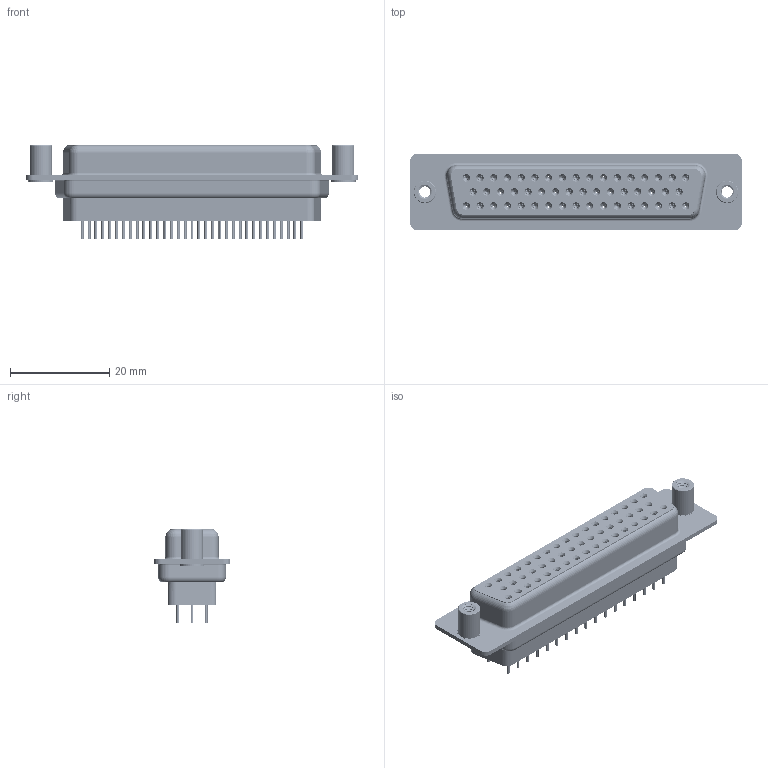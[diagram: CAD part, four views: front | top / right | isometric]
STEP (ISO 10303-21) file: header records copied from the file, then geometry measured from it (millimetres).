
FILE_DESCRIPTION (( 'STEP AP203' ), '1' );
FILE_NAME ('628-050-228-268.STEP', '2020-07-21T01:35:46', ( '' ), ( '' ), 'SwSTEP 2.0', 'SolidWorks 2020', '' );
FILE_SCHEMA (( 'CONFIG_CONTROL_DESIGN' ));
Length unit declared in the file: millimetre
Products named in the file (8): 628 4-40 Threaded Standoff; 628 Contact Row 1_28L; 628 Housing_50 FF; 628 Contact Row 2_28L; 628 Shell Front_50 Contacts; 628 Shell Rear_50 Contacts; 628-050-228-268; 628 Contact Row 3_28L
Assembly tree (55 placements, depth 2):
  628-050-228-268
    628 Housing_50 FF
    628 Shell Front_50 Contacts
    628 Shell Rear_50 Contacts
    628 Contact Row 1_28L  x17
    628 Contact Row 2_28L  x16
    628 Contact Row 3_28L  x17
    628 4-40 Threaded Standoff  x2
Bounding box: 67 x 15.4 x 18.8 mm (x, y, z)
Volume: 7912.8 mm3; surface area: 17630.9 mm2
Topology: 56 solids, 56 shells, 6774 faces, 17306 edges, 10757 vertices
Faces by surface type: cylinder 1920, plane 1625, torus 1363, bspline 1006, cone 860
Entity records: 47071 total; most frequent: CARTESIAN_POINT 12265, DIRECTION 7276, ORIENTED_EDGE 6502, EDGE_CURVE 3251, AXIS2_PLACEMENT_3D 3070, VERTEX_POINT 2067, EDGE_LOOP 1734, CIRCLE 1715
